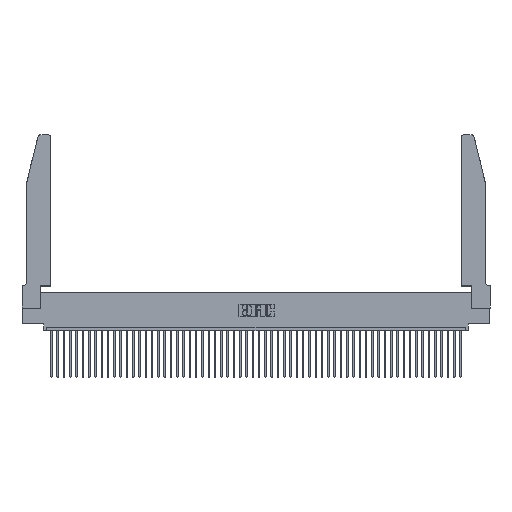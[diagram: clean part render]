
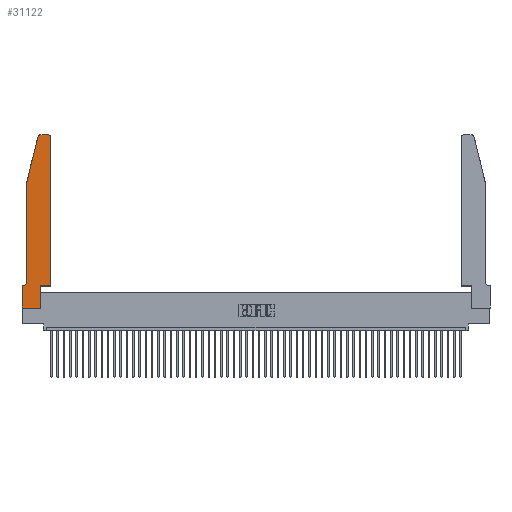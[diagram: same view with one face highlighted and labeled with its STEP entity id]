
A CAD part, top view. The second image highlights one B-rep face of the part: STEP entity #31122.
In plain terms, the highlighted planar face has unit normal (0, 0, 1).
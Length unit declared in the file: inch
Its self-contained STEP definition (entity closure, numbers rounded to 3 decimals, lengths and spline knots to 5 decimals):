
#393 = AXIS2_PLACEMENT_3D ( 'NONE', #6421, #50697, #11072 ) ;
#2452 = VECTOR ( 'NONE', #50143, 39.37008 ) ;
#3389 = DIRECTION ( 'NONE',  ( 0., -1., 0. ) ) ;
#3666 = CARTESIAN_POINT ( 'NONE',  ( 0.2605, 2.75, 0.37 ) ) ;
#3828 = DIRECTION ( 'NONE',  ( 1., 0., 0. ) ) ;
#4045 = VERTEX_POINT ( 'NONE', #30307 ) ;
#4047 = DIRECTION ( 'NONE',  ( 0., 0., 1. ) ) ;
#4166 = PLANE ( 'NONE',  #44357 ) ;
#4366 = EDGE_CURVE ( 'NONE', #46253, #15553, #8553, .T. ) ;
#4369 = LINE ( 'NONE', #35545, #7525 ) ;
#4512 = CARTESIAN_POINT ( 'NONE',  ( 0.4205, 2.72, 0.37 ) ) ;
#4541 = VERTEX_POINT ( 'NONE', #19159 ) ;
#4806 = CIRCLE ( 'NONE', #25318, 0.03 ) ;
#6299 = VERTEX_POINT ( 'NONE', #37508 ) ;
#6421 = CARTESIAN_POINT ( 'NONE',  ( 0.0055, 0.42, 0.37 ) ) ;
#6683 = LINE ( 'NONE', #23795, #17092 ) ;
#6903 = CIRCLE ( 'NONE', #393, 0.07 ) ;
#7383 = LINE ( 'NONE', #15735, #47676 ) ;
#7525 = VECTOR ( 'NONE', #28187, 39.37008 ) ;
#8092 = VERTEX_POINT ( 'NONE', #45195 ) ;
#8345 = VERTEX_POINT ( 'NONE', #50651 ) ;
#8527 = EDGE_CURVE ( 'NONE', #15553, #16403, #45332, .T. ) ;
#8553 = LINE ( 'NONE', #42268, #31494 ) ;
#8932 = CARTESIAN_POINT ( 'NONE',  ( 0.2865, 0., 0.37 ) ) ;
#9321 = DIRECTION ( 'NONE',  ( 0., 0., 1. ) ) ;
#9745 = ORIENTED_EDGE ( 'NONE', *, *, #13909, .T. ) ;
#10605 = EDGE_LOOP ( 'NONE', ( #9745, #36405, #29542, #45913, #28900, #46801, #13979, #28230, #30202, #38396, #23134, #48486 ) ) ;
#10658 = EDGE_CURVE ( 'NONE', #16403, #8092, #4369, .T. ) ;
#11072 = DIRECTION ( 'NONE',  ( -1., 0., 0. ) ) ;
#11180 = AXIS2_PLACEMENT_3D ( 'NONE', #4512, #9321, #49606 ) ;
#11724 = CARTESIAN_POINT ( 'NONE',  ( 0., 0.35, 0.37 ) ) ;
#12474 = EDGE_CURVE ( 'NONE', #4045, #4541, #24485, .T. ) ;
#13909 = EDGE_CURVE ( 'NONE', #4541, #8345, #22613, .T. ) ;
#13979 = ORIENTED_EDGE ( 'NONE', *, *, #45333, .T. ) ;
#14221 = CARTESIAN_POINT ( 'NONE',  ( 0.0755, 0.42, 0.37 ) ) ;
#15553 = VERTEX_POINT ( 'NONE', #8932 ) ;
#15735 = CARTESIAN_POINT ( 'NONE',  ( 0., 0., 0.37 ) ) ;
#16403 = VERTEX_POINT ( 'NONE', #46528 ) ;
#17092 = VECTOR ( 'NONE', #39839, 39.37008 ) ;
#17436 = CARTESIAN_POINT ( 'NONE',  ( 0.0055, 0.35, 0.37 ) ) ;
#19011 = EDGE_CURVE ( 'NONE', #8092, #4045, #35089, .T. ) ;
#19159 = CARTESIAN_POINT ( 'NONE',  ( 0.4205, 2.75, 0.37 ) ) ;
#22047 = CARTESIAN_POINT ( 'NONE',  ( 0., 0., 0.37 ) ) ;
#22613 = LINE ( 'NONE', #3666, #41955 ) ;
#22621 = VECTOR ( 'NONE', #28146, 39.37008 ) ;
#23134 = ORIENTED_EDGE ( 'NONE', *, *, #19011, .T. ) ;
#23162 = DIRECTION ( 'NONE',  ( -1., 0., 0. ) ) ;
#23496 = DIRECTION ( 'NONE',  ( 0., 0., 1. ) ) ;
#23795 = CARTESIAN_POINT ( 'NONE',  ( 0.0755, 2., 0.37 ) ) ;
#24347 = LINE ( 'NONE', #49274, #36872 ) ;
#24485 = CIRCLE ( 'NONE', #11180, 0.03 ) ;
#25318 = AXIS2_PLACEMENT_3D ( 'NONE', #47432, #4047, #35594 ) ;
#25406 = DIRECTION ( 'NONE',  ( -1., 0., 0. ) ) ;
#25410 = FACE_OUTER_BOUND ( 'NONE', #10605, .T. ) ;
#27103 = EDGE_CURVE ( 'NONE', #35783, #50729, #6683, .T. ) ;
#28146 = DIRECTION ( 'NONE',  ( 0., 1., 0. ) ) ;
#28187 = DIRECTION ( 'NONE',  ( 1., 0., 0. ) ) ;
#28230 = ORIENTED_EDGE ( 'NONE', *, *, #4366, .T. ) ;
#28900 = ORIENTED_EDGE ( 'NONE', *, *, #39751, .T. ) ;
#29542 = ORIENTED_EDGE ( 'NONE', *, *, #32023, .T. ) ;
#30202 = ORIENTED_EDGE ( 'NONE', *, *, #8527, .T. ) ;
#30307 = CARTESIAN_POINT ( 'NONE',  ( 0.4505, 2.72, 0.37 ) ) ;
#31122 = ADVANCED_FACE ( 'NONE', ( #25410 ), #4166, .T. ) ;
#31372 = CARTESIAN_POINT ( 'NONE',  ( 0., 0.35, 0.37 ) ) ;
#31494 = VECTOR ( 'NONE', #43487, 39.37008 ) ;
#32023 = EDGE_CURVE ( 'NONE', #6299, #35783, #47164, .T. ) ;
#32933 = EDGE_CURVE ( 'NONE', #8345, #6299, #4806, .T. ) ;
#34455 = CARTESIAN_POINT ( 'NONE',  ( 0.0755, 2., 0.37 ) ) ;
#35089 = LINE ( 'NONE', #36495, #22621 ) ;
#35456 = CARTESIAN_POINT ( 'NONE',  ( 0.0755, 2., 0.37 ) ) ;
#35545 = CARTESIAN_POINT ( 'NONE',  ( 0.4505, 0.35, 0.37 ) ) ;
#35594 = DIRECTION ( 'NONE',  ( 1., 0., 0. ) ) ;
#35783 = VERTEX_POINT ( 'NONE', #35456 ) ;
#36405 = ORIENTED_EDGE ( 'NONE', *, *, #32933, .T. ) ;
#36495 = CARTESIAN_POINT ( 'NONE',  ( 0.4505, 0.35, 0.37 ) ) ;
#36604 = EDGE_CURVE ( 'NONE', #48066, #39952, #24347, .T. ) ;
#36872 = VECTOR ( 'NONE', #25406, 39.37008 ) ;
#37508 = CARTESIAN_POINT ( 'NONE',  ( 0.25487, 2.72718, 0.37 ) ) ;
#38396 = ORIENTED_EDGE ( 'NONE', *, *, #10658, .T. ) ;
#39751 = EDGE_CURVE ( 'NONE', #50729, #48066, #6903, .T. ) ;
#39839 = DIRECTION ( 'NONE',  ( 0., -1., 0. ) ) ;
#39952 = VERTEX_POINT ( 'NONE', #11724 ) ;
#41955 = VECTOR ( 'NONE', #23162, 39.37008 ) ;
#41969 = CARTESIAN_POINT ( 'NONE',  ( 0.2865, 0.35, 0.37 ) ) ;
#42268 = CARTESIAN_POINT ( 'NONE',  ( 0., 0., 0.37 ) ) ;
#43487 = DIRECTION ( 'NONE',  ( 1., 0., 0. ) ) ;
#44357 = AXIS2_PLACEMENT_3D ( 'NONE', #31372, #23496, #3828 ) ;
#45195 = CARTESIAN_POINT ( 'NONE',  ( 0.4505, 0.35, 0.37 ) ) ;
#45332 = LINE ( 'NONE', #41969, #49657 ) ;
#45333 = EDGE_CURVE ( 'NONE', #39952, #46253, #7383, .T. ) ;
#45913 = ORIENTED_EDGE ( 'NONE', *, *, #27103, .T. ) ;
#46253 = VERTEX_POINT ( 'NONE', #22047 ) ;
#46528 = CARTESIAN_POINT ( 'NONE',  ( 0.2865, 0.35, 0.37 ) ) ;
#46801 = ORIENTED_EDGE ( 'NONE', *, *, #36604, .T. ) ;
#47164 = LINE ( 'NONE', #34455, #2452 ) ;
#47432 = CARTESIAN_POINT ( 'NONE',  ( 0.284, 2.72, 0.37 ) ) ;
#47676 = VECTOR ( 'NONE', #3389, 39.37008 ) ;
#48066 = VERTEX_POINT ( 'NONE', #17436 ) ;
#48486 = ORIENTED_EDGE ( 'NONE', *, *, #12474, .T. ) ;
#49274 = CARTESIAN_POINT ( 'NONE',  ( 0.0755, 0.35, 0.37 ) ) ;
#49445 = DIRECTION ( 'NONE',  ( 0., 1., 0. ) ) ;
#49606 = DIRECTION ( 'NONE',  ( 1., 0., 0. ) ) ;
#49657 = VECTOR ( 'NONE', #49445, 39.37008 ) ;
#50143 = DIRECTION ( 'NONE',  ( -0.239, -0.971, 0. ) ) ;
#50651 = CARTESIAN_POINT ( 'NONE',  ( 0.284, 2.75, 0.37 ) ) ;
#50697 = DIRECTION ( 'NONE',  ( 0., 0., -1. ) ) ;
#50729 = VERTEX_POINT ( 'NONE', #14221 ) ;
